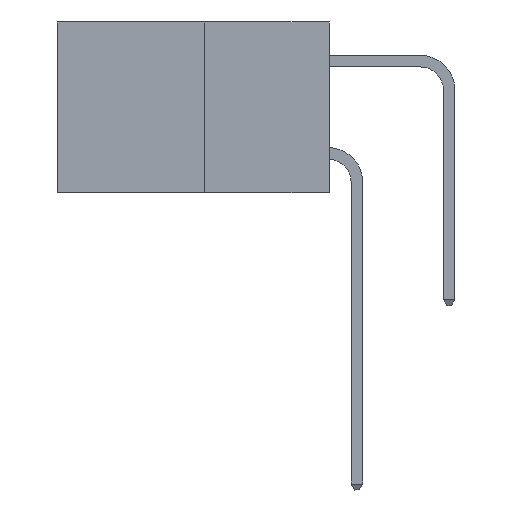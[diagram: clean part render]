
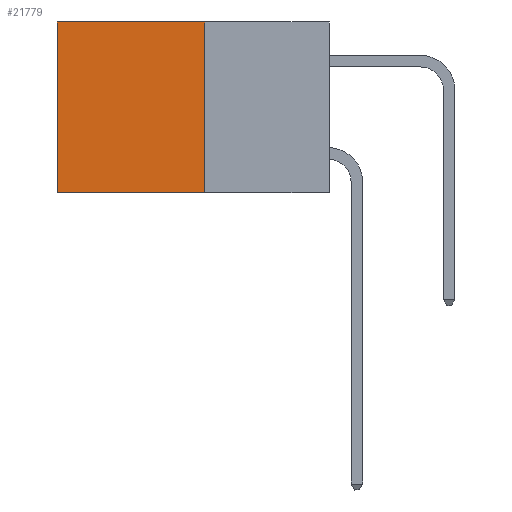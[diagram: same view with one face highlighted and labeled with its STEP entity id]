
A CAD part, left-side view. The second image highlights one B-rep face of the part: STEP entity #21779.
In plain terms, the highlighted planar face has unit normal (-1, 0, 0).
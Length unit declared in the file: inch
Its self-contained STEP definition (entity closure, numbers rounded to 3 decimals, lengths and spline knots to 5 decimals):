
#753 = EDGE_CURVE ( 'NONE', #14043, #9759, #3786, .T. ) ;
#2348 = ORIENTED_EDGE ( 'NONE', *, *, #753, .T. ) ;
#2890 = VERTEX_POINT ( 'NONE', #5293 ) ;
#2894 = VECTOR ( 'NONE', #15503, 39.37008 ) ;
#3140 = AXIS2_PLACEMENT_3D ( 'NONE', #7192, #9415, #24594 ) ;
#3222 = CARTESIAN_POINT ( 'NONE',  ( 0.277, 0.59, -0.37 ) ) ;
#3314 = EDGE_LOOP ( 'NONE', ( #27677, #21463, #19519, #2348 ) ) ;
#3536 = VECTOR ( 'NONE', #12094, 39.37008 ) ;
#3722 = LINE ( 'NONE', #16582, #19904 ) ;
#3786 = LINE ( 'NONE', #6855, #14909 ) ;
#5293 = CARTESIAN_POINT ( 'NONE',  ( 0.277, 0.27, -0.37 ) ) ;
#5786 = CARTESIAN_POINT ( 'NONE',  ( 0.277, 0.27, 0. ) ) ;
#5980 = FACE_OUTER_BOUND ( 'NONE', #3314, .T. ) ;
#6855 = CARTESIAN_POINT ( 'NONE',  ( 0.277, 0.27, 0. ) ) ;
#7192 = CARTESIAN_POINT ( 'NONE',  ( 0.277, 0.27, -0.37 ) ) ;
#7346 = DIRECTION ( 'NONE',  ( 0., 1., 0. ) ) ;
#7833 = DIRECTION ( 'NONE',  ( 0., 1., 0. ) ) ;
#9415 = DIRECTION ( 'NONE',  ( 1., 0., 0. ) ) ;
#9759 = VERTEX_POINT ( 'NONE', #12936 ) ;
#12094 = DIRECTION ( 'NONE',  ( 0., 0., -1. ) ) ;
#12258 = CARTESIAN_POINT ( 'NONE',  ( 0.277, 0.59, -0.37 ) ) ;
#12936 = CARTESIAN_POINT ( 'NONE',  ( 0.277, 0.59, 0. ) ) ;
#14043 = VERTEX_POINT ( 'NONE', #5786 ) ;
#14909 = VECTOR ( 'NONE', #7346, 39.37008 ) ;
#15503 = DIRECTION ( 'NONE',  ( 0., 0., -1. ) ) ;
#16582 = CARTESIAN_POINT ( 'NONE',  ( 0.277, 0.27, -0.37 ) ) ;
#18484 = VERTEX_POINT ( 'NONE', #12258 ) ;
#18772 = EDGE_CURVE ( 'NONE', #14043, #2890, #26190, .T. ) ;
#19519 = ORIENTED_EDGE ( 'NONE', *, *, #18772, .F. ) ;
#19904 = VECTOR ( 'NONE', #7833, 39.37008 ) ;
#20258 = PLANE ( 'NONE',  #3140 ) ;
#21463 = ORIENTED_EDGE ( 'NONE', *, *, #27527, .F. ) ;
#21719 = LINE ( 'NONE', #3222, #3536 ) ;
#21779 = ADVANCED_FACE ( 'NONE', ( #5980 ), #20258, .F. ) ;
#24072 = CARTESIAN_POINT ( 'NONE',  ( 0.277, 0.27, -0.37 ) ) ;
#24594 = DIRECTION ( 'NONE',  ( 0., 0., -1. ) ) ;
#25088 = EDGE_CURVE ( 'NONE', #9759, #18484, #21719, .T. ) ;
#26190 = LINE ( 'NONE', #24072, #2894 ) ;
#27527 = EDGE_CURVE ( 'NONE', #2890, #18484, #3722, .T. ) ;
#27677 = ORIENTED_EDGE ( 'NONE', *, *, #25088, .T. ) ;
